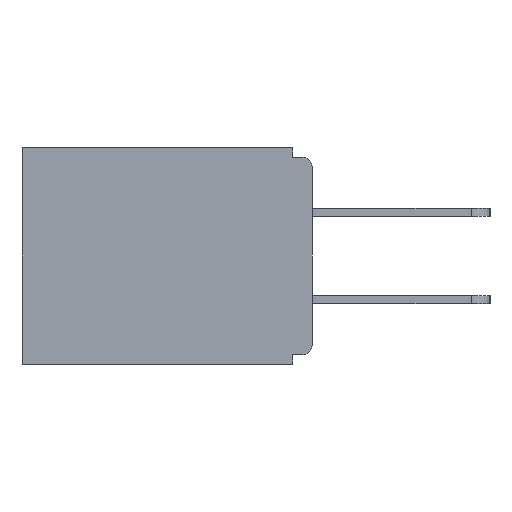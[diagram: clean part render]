
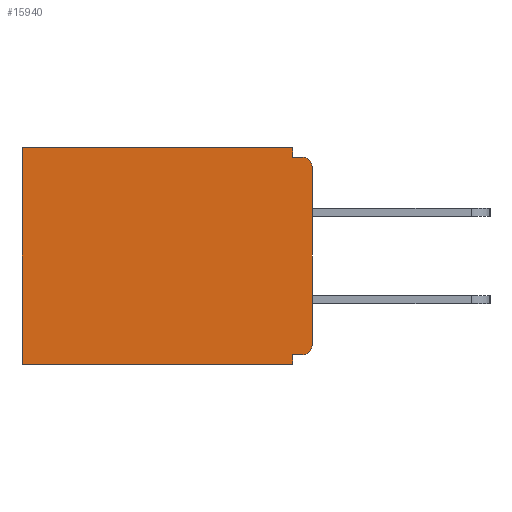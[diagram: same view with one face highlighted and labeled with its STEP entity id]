
A CAD part, left-side view. The second image highlights one B-rep face of the part: STEP entity #15940.
In plain terms, the highlighted planar face has unit normal (-1, 0, 0).
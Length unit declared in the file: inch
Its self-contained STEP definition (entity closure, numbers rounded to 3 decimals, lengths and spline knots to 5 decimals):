
#81 = AXIS2_PLACEMENT_3D ( 'NONE', #19797, #20022, #5119 ) ;
#193 = VECTOR ( 'NONE', #11476, 39.37008 ) ;
#508 = VECTOR ( 'NONE', #3113, 39.37008 ) ;
#744 = FACE_OUTER_BOUND ( 'NONE', #3085, .T. ) ;
#841 = DIRECTION ( 'NONE',  ( 0., 0., -1. ) ) ;
#968 = EDGE_CURVE ( 'NONE', #13755, #9748, #12695, .T. ) ;
#1425 = EDGE_CURVE ( 'NONE', #14656, #15909, #14483, .T. ) ;
#1454 = VECTOR ( 'NONE', #841, 39.37008 ) ;
#1457 = CARTESIAN_POINT ( 'NONE',  ( 0.298, 0.031, -0.343 ) ) ;
#1503 = ORIENTED_EDGE ( 'NONE', *, *, #13720, .F. ) ;
#1827 = VECTOR ( 'NONE', #15095, 39.37008 ) ;
#1839 = VECTOR ( 'NONE', #5964, 39.37008 ) ;
#2280 = CARTESIAN_POINT ( 'NONE',  ( 0.298, 0., 0. ) ) ;
#2326 = VERTEX_POINT ( 'NONE', #8706 ) ;
#2426 = DIRECTION ( 'NONE',  ( 1., 0., 0. ) ) ;
#2502 = EDGE_CURVE ( 'NONE', #13071, #2326, #8835, .T. ) ;
#2554 = EDGE_CURVE ( 'NONE', #3711, #5837, #14450, .T. ) ;
#2754 = ORIENTED_EDGE ( 'NONE', *, *, #16244, .T. ) ;
#3085 = EDGE_LOOP ( 'NONE', ( #6103, #1503, #4197, #16068, #10973, #9199, #8185, #11305, #2754, #17773 ) ) ;
#3113 = DIRECTION ( 'NONE',  ( 0., 0., -1. ) ) ;
#3168 = CIRCLE ( 'NONE', #81, 0.015 ) ;
#3366 = CARTESIAN_POINT ( 'NONE',  ( 0.298, 0.031, -0.343 ) ) ;
#3546 = LINE ( 'NONE', #8213, #15538 ) ;
#3711 = VERTEX_POINT ( 'NONE', #7116 ) ;
#4007 = VECTOR ( 'NONE', #5280, 39.37008 ) ;
#4197 = ORIENTED_EDGE ( 'NONE', *, *, #968, .F. ) ;
#4280 = CARTESIAN_POINT ( 'NONE',  ( 0.298, 0.015, -0.328 ) ) ;
#4839 = LINE ( 'NONE', #1457, #508 ) ;
#5119 = DIRECTION ( 'NONE',  ( 0., 0., -1. ) ) ;
#5280 = DIRECTION ( 'NONE',  ( 0., 1., 0. ) ) ;
#5837 = VERTEX_POINT ( 'NONE', #15556 ) ;
#5906 = CARTESIAN_POINT ( 'NONE',  ( 0.298, 0., -0.03 ) ) ;
#5964 = DIRECTION ( 'NONE',  ( 0., 1., 0. ) ) ;
#6103 = ORIENTED_EDGE ( 'NONE', *, *, #12428, .T. ) ;
#7116 = CARTESIAN_POINT ( 'NONE',  ( 0.298, 0.46, 0. ) ) ;
#7340 = PLANE ( 'NONE',  #20153 ) ;
#7932 = LINE ( 'NONE', #8508, #1827 ) ;
#8185 = ORIENTED_EDGE ( 'NONE', *, *, #17039, .F. ) ;
#8211 = LINE ( 'NONE', #14085, #1839 ) ;
#8213 = CARTESIAN_POINT ( 'NONE',  ( 0.298, 0., 0. ) ) ;
#8402 = CARTESIAN_POINT ( 'NONE',  ( 0.298, 0.031, -0.343 ) ) ;
#8508 = CARTESIAN_POINT ( 'NONE',  ( 0.298, 0., -0.015 ) ) ;
#8626 = CARTESIAN_POINT ( 'NONE',  ( 0.298, 0.46, 0. ) ) ;
#8706 = CARTESIAN_POINT ( 'NONE',  ( 0.298, 0.031, -0.328 ) ) ;
#8773 = CARTESIAN_POINT ( 'NONE',  ( 0.298, 0., -0.328 ) ) ;
#8799 = CARTESIAN_POINT ( 'NONE',  ( 0.298, 0.031, -0.015 ) ) ;
#8835 = LINE ( 'NONE', #8773, #4007 ) ;
#8908 = CARTESIAN_POINT ( 'NONE',  ( 0.298, 0.015, -0.015 ) ) ;
#9072 = DIRECTION ( 'NONE',  ( -1., 0., 0. ) ) ;
#9199 = ORIENTED_EDGE ( 'NONE', *, *, #9767, .F. ) ;
#9748 = VERTEX_POINT ( 'NONE', #8799 ) ;
#9767 = EDGE_CURVE ( 'NONE', #18112, #5837, #8211, .T. ) ;
#10157 = CIRCLE ( 'NONE', #13393, 0.015 ) ;
#10346 = CARTESIAN_POINT ( 'NONE',  ( 0.298, 0., -0.313 ) ) ;
#10531 = CARTESIAN_POINT ( 'NONE',  ( 0.298, 0., 0. ) ) ;
#10548 = DIRECTION ( 'NONE',  ( 0., 0., -1. ) ) ;
#10973 = ORIENTED_EDGE ( 'NONE', *, *, #2554, .T. ) ;
#11305 = ORIENTED_EDGE ( 'NONE', *, *, #2502, .F. ) ;
#11476 = DIRECTION ( 'NONE',  ( 0., 0., -1. ) ) ;
#11649 = DIRECTION ( 'NONE',  ( 0., 1., 0. ) ) ;
#11995 = EDGE_CURVE ( 'NONE', #13755, #3711, #3546, .T. ) ;
#12428 = EDGE_CURVE ( 'NONE', #14656, #17515, #3168, .T. ) ;
#12695 = LINE ( 'NONE', #3366, #193 ) ;
#13071 = VERTEX_POINT ( 'NONE', #4280 ) ;
#13393 = AXIS2_PLACEMENT_3D ( 'NONE', #18892, #9072, #18961 ) ;
#13720 = EDGE_CURVE ( 'NONE', #9748, #17515, #7932, .T. ) ;
#13755 = VERTEX_POINT ( 'NONE', #18462 ) ;
#14085 = CARTESIAN_POINT ( 'NONE',  ( 0.298, 0., -0.343 ) ) ;
#14450 = LINE ( 'NONE', #8626, #15774 ) ;
#14483 = LINE ( 'NONE', #10531, #1454 ) ;
#14656 = VERTEX_POINT ( 'NONE', #5906 ) ;
#15095 = DIRECTION ( 'NONE',  ( 0., -1., 0. ) ) ;
#15538 = VECTOR ( 'NONE', #11649, 39.37008 ) ;
#15556 = CARTESIAN_POINT ( 'NONE',  ( 0.298, 0.46, -0.343 ) ) ;
#15774 = VECTOR ( 'NONE', #16642, 39.37008 ) ;
#15909 = VERTEX_POINT ( 'NONE', #10346 ) ;
#15940 = ADVANCED_FACE ( 'NONE', ( #744 ), #7340, .F. ) ;
#16068 = ORIENTED_EDGE ( 'NONE', *, *, #11995, .T. ) ;
#16244 = EDGE_CURVE ( 'NONE', #13071, #15909, #10157, .T. ) ;
#16642 = DIRECTION ( 'NONE',  ( 0., 0., -1. ) ) ;
#17039 = EDGE_CURVE ( 'NONE', #2326, #18112, #4839, .T. ) ;
#17515 = VERTEX_POINT ( 'NONE', #8908 ) ;
#17773 = ORIENTED_EDGE ( 'NONE', *, *, #1425, .F. ) ;
#18112 = VERTEX_POINT ( 'NONE', #8402 ) ;
#18462 = CARTESIAN_POINT ( 'NONE',  ( 0.298, 0.031, 0. ) ) ;
#18892 = CARTESIAN_POINT ( 'NONE',  ( 0.298, 0.015, -0.313 ) ) ;
#18961 = DIRECTION ( 'NONE',  ( 0., 0., -1. ) ) ;
#19797 = CARTESIAN_POINT ( 'NONE',  ( 0.298, 0.015, -0.03 ) ) ;
#20022 = DIRECTION ( 'NONE',  ( -1., 0., 0. ) ) ;
#20153 = AXIS2_PLACEMENT_3D ( 'NONE', #2280, #2426, #10548 ) ;
